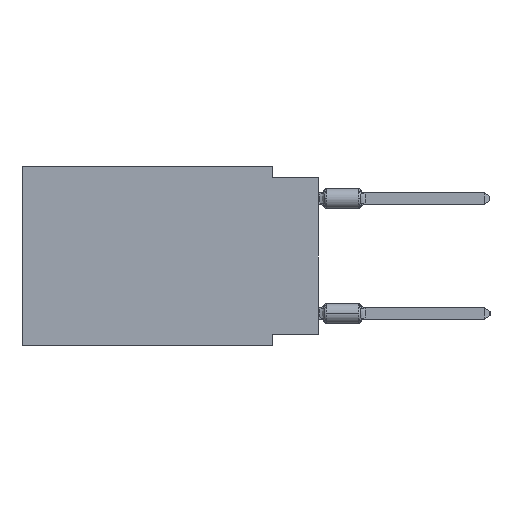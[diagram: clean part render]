
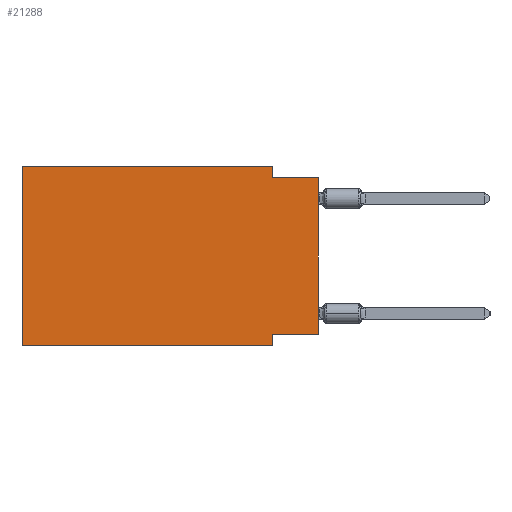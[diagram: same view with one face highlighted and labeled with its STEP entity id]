
A CAD part, left-side view. The second image highlights one B-rep face of the part: STEP entity #21288.
In plain terms, the highlighted planar face has unit normal (-1, 0, 0).
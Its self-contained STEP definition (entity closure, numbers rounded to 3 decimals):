
#2479 = VECTOR ( 'NONE', #27294, 1000. ) ;
#3399 = VECTOR ( 'NONE', #29471, 1000. ) ;
#4441 = LINE ( 'NONE', #15021, #41813 ) ;
#4529 = CARTESIAN_POINT ( 'NONE',  ( 0., 16.383, 0. ) ) ;
#4692 = LINE ( 'NONE', #14303, #54735 ) ;
#5297 = VERTEX_POINT ( 'NONE', #28286 ) ;
#5912 = LINE ( 'NONE', #11043, #39586 ) ;
#7115 = CARTESIAN_POINT ( 'NONE',  ( 0., 0., -9.271 ) ) ;
#7418 = CARTESIAN_POINT ( 'NONE',  ( 0., 2.54, -9.906 ) ) ;
#8235 = AXIS2_PLACEMENT_3D ( 'NONE', #57068, #37500, #22719 ) ;
#8384 = VERTEX_POINT ( 'NONE', #30131 ) ;
#8735 = VERTEX_POINT ( 'NONE', #49634 ) ;
#9359 = VERTEX_POINT ( 'NONE', #36677 ) ;
#9493 = DIRECTION ( 'NONE',  ( 0., 0., -1. ) ) ;
#11043 = CARTESIAN_POINT ( 'NONE',  ( 0., 2.54, 0. ) ) ;
#11346 = DIRECTION ( 'NONE',  ( 0., 0., -1. ) ) ;
#11621 = LINE ( 'NONE', #7115, #25967 ) ;
#11694 = EDGE_CURVE ( 'NONE', #8735, #42534, #11621, .T. ) ;
#12656 = ORIENTED_EDGE ( 'NONE', *, *, #16631, .T. ) ;
#12921 = EDGE_LOOP ( 'NONE', ( #12656, #58194, #60302, #56178, #35362, #37801, #18015, #60364 ) ) ;
#14303 = CARTESIAN_POINT ( 'NONE',  ( 0., 2.54, -9.906 ) ) ;
#14610 = EDGE_CURVE ( 'NONE', #8384, #23561, #5912, .T. ) ;
#15021 = CARTESIAN_POINT ( 'NONE',  ( 0., 0., 0. ) ) ;
#16631 = EDGE_CURVE ( 'NONE', #8735, #9359, #4441, .T. ) ;
#16674 = CARTESIAN_POINT ( 'NONE',  ( 0., 16.383, 0. ) ) ;
#17663 = CARTESIAN_POINT ( 'NONE',  ( 0., 16.383, 0. ) ) ;
#18015 = ORIENTED_EDGE ( 'NONE', *, *, #41139, .F. ) ;
#18610 = LINE ( 'NONE', #17663, #2479 ) ;
#21194 = DIRECTION ( 'NONE',  ( 0., -1., 0. ) ) ;
#21288 = ADVANCED_FACE ( 'NONE', ( #27854 ), #28817, .F. ) ;
#22719 = DIRECTION ( 'NONE',  ( 0., 0., -1. ) ) ;
#23364 = LINE ( 'NONE', #24640, #3399 ) ;
#23561 = VERTEX_POINT ( 'NONE', #33712 ) ;
#23824 = CARTESIAN_POINT ( 'NONE',  ( 0., 2.54, -9.271 ) ) ;
#24640 = CARTESIAN_POINT ( 'NONE',  ( 0., 0., -0.635 ) ) ;
#25967 = VECTOR ( 'NONE', #40846, 1000. ) ;
#26605 = LINE ( 'NONE', #16674, #60224 ) ;
#27294 = DIRECTION ( 'NONE',  ( 0., 0., 1. ) ) ;
#27854 = FACE_OUTER_BOUND ( 'NONE', #12921, .T. ) ;
#28286 = CARTESIAN_POINT ( 'NONE',  ( 0., 16.383, -9.906 ) ) ;
#28817 = PLANE ( 'NONE',  #8235 ) ;
#29471 = DIRECTION ( 'NONE',  ( 0., -1., 0. ) ) ;
#30131 = CARTESIAN_POINT ( 'NONE',  ( 0., 2.54, 0. ) ) ;
#31705 = EDGE_CURVE ( 'NONE', #5297, #46803, #18610, .T. ) ;
#32639 = LINE ( 'NONE', #56698, #54140 ) ;
#33712 = CARTESIAN_POINT ( 'NONE',  ( 0., 2.54, -0.635 ) ) ;
#35362 = ORIENTED_EDGE ( 'NONE', *, *, #31705, .F. ) ;
#36677 = CARTESIAN_POINT ( 'NONE',  ( 0., 0., -0.635 ) ) ;
#37094 = EDGE_CURVE ( 'NONE', #46803, #8384, #26605, .T. ) ;
#37500 = DIRECTION ( 'NONE',  ( 1., 0., 0. ) ) ;
#37801 = ORIENTED_EDGE ( 'NONE', *, *, #49015, .T. ) ;
#39416 = DIRECTION ( 'NONE',  ( 0., 0., 1. ) ) ;
#39586 = VECTOR ( 'NONE', #11346, 1000. ) ;
#40778 = EDGE_CURVE ( 'NONE', #23561, #9359, #23364, .T. ) ;
#40846 = DIRECTION ( 'NONE',  ( 0., 1., 0. ) ) ;
#41139 = EDGE_CURVE ( 'NONE', #42534, #58320, #4692, .T. ) ;
#41813 = VECTOR ( 'NONE', #39416, 1000. ) ;
#42534 = VERTEX_POINT ( 'NONE', #23824 ) ;
#46803 = VERTEX_POINT ( 'NONE', #4529 ) ;
#49015 = EDGE_CURVE ( 'NONE', #5297, #58320, #32639, .T. ) ;
#49634 = CARTESIAN_POINT ( 'NONE',  ( 0., 0., -9.271 ) ) ;
#52204 = DIRECTION ( 'NONE',  ( 0., -1., 0. ) ) ;
#54140 = VECTOR ( 'NONE', #52204, 1000. ) ;
#54735 = VECTOR ( 'NONE', #9493, 1000. ) ;
#56178 = ORIENTED_EDGE ( 'NONE', *, *, #37094, .F. ) ;
#56698 = CARTESIAN_POINT ( 'NONE',  ( 0., 16.383, -9.906 ) ) ;
#57068 = CARTESIAN_POINT ( 'NONE',  ( 0., 16.383, 0. ) ) ;
#58194 = ORIENTED_EDGE ( 'NONE', *, *, #40778, .F. ) ;
#58320 = VERTEX_POINT ( 'NONE', #7418 ) ;
#60224 = VECTOR ( 'NONE', #21194, 1000. ) ;
#60302 = ORIENTED_EDGE ( 'NONE', *, *, #14610, .F. ) ;
#60364 = ORIENTED_EDGE ( 'NONE', *, *, #11694, .F. ) ;
